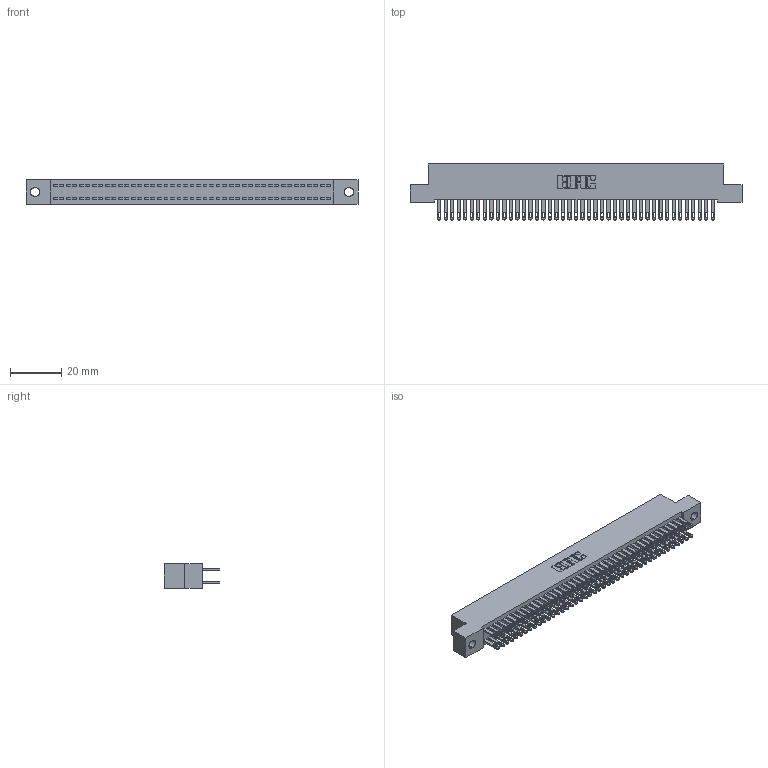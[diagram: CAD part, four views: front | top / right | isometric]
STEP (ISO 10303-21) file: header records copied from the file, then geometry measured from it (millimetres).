
FILE_DESCRIPTION (( 'STEP AP203' ), '1' );
FILE_NAME ('892-086-500-202.STEP', '2020-09-21T20:29:52', ( '' ), ( '' ), 'SwSTEP 2.0', 'SolidWorks 2020', '' );
FILE_SCHEMA (( 'CONFIG_CONTROL_DESIGN' ));
Length unit declared in the file: inch
Products named in the file (3): 842 Part_.128 Slot; 892-086-500-202; 345-292-001_345-293-100
Assembly tree (87 placements, depth 2):
  892-086-500-202
    842 Part_.128 Slot
    345-292-001_345-293-100  x86
Bounding box: 129.54 x 21.85 x 9.4 mm (x, y, z)
Volume: 11854.5 mm3; surface area: 19903.7 mm2
Topology: 87 solids, 87 shells, 4242 faces, 12953 edges, 8634 vertices
Faces by surface type: plane 2650, cylinder 1592
Entity records: 27467 total; most frequent: CARTESIAN_POINT 4550, ORIENTED_EDGE 4486, DIRECTION 3887, EDGE_CURVE 2243, LINE 2111, VECTOR 2111, VERTEX_POINT 1494, AXIS2_PLACEMENT_3D 888
